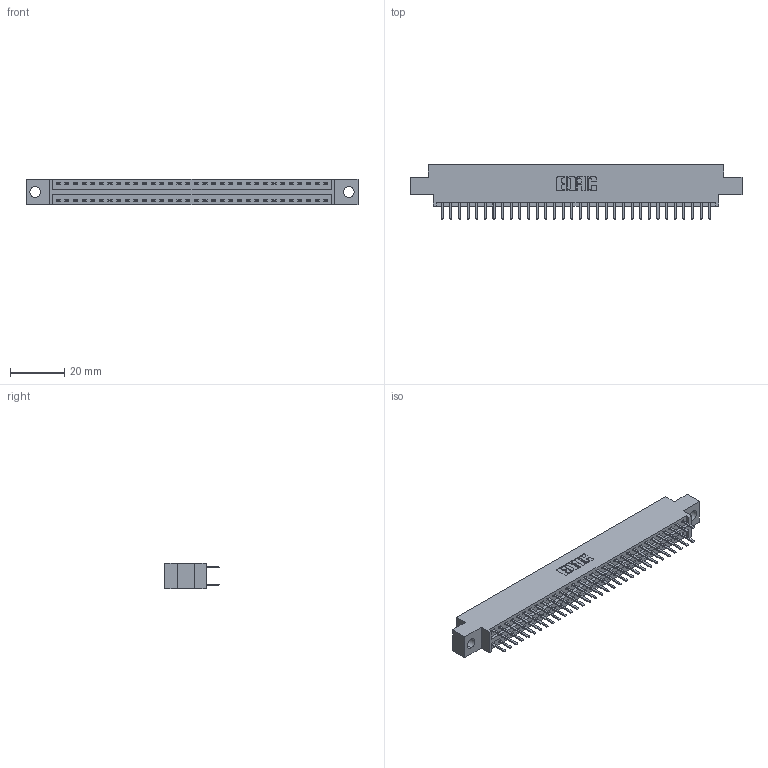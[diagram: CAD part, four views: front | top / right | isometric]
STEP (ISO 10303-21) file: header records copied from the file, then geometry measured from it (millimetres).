
FILE_DESCRIPTION (( 'STEP AP203' ), '1' );
FILE_NAME ('346-064-520-804.STEP', '2022-05-24T14:55:03', ( '' ), ( '' ), 'SwSTEP 2.0', 'SolidWorks 2020', '' );
FILE_SCHEMA (( 'CONFIG_CONTROL_DESIGN' ));
Length unit declared in the file: inch
Products named in the file (3): 346 Part_0.170 Offset - 0.156 Dia-TH; 346-064-520-804; 345-292-001_345-293-120
Assembly tree (65 placements, depth 2):
  346-064-520-804
    346 Part_0.170 Offset - 0.156 Dia-TH
    345-292-001_345-293-120  x64
Bounding box: 122.17 x 20.02 x 9.4 mm (x, y, z)
Volume: 11547.1 mm3; surface area: 15676.7 mm2
Topology: 65 solids, 65 shells, 3724 faces, 10809 edges, 7034 vertices
Faces by surface type: plane 2462, cylinder 1262
Entity records: 22895 total; most frequent: CARTESIAN_POINT 3806, ORIENTED_EDGE 3726, DIRECTION 3391, EDGE_CURVE 1863, VECTOR 1599, LINE 1599, VERTEX_POINT 1238, AXIS2_PLACEMENT_3D 896
